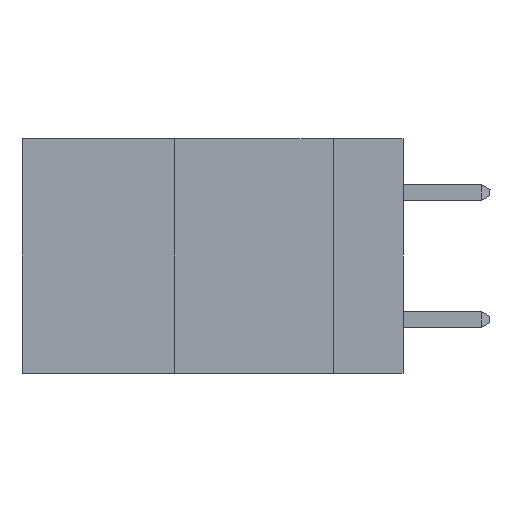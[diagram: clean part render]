
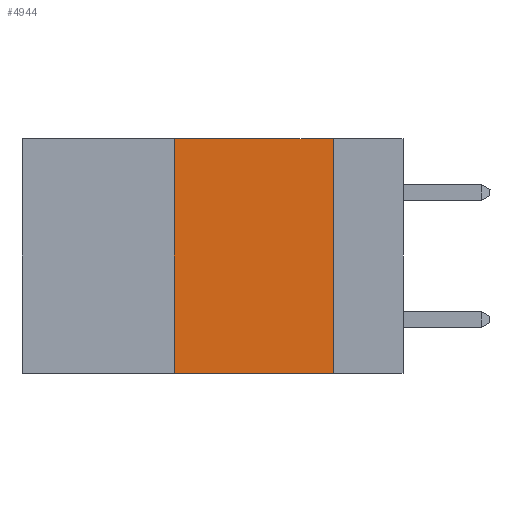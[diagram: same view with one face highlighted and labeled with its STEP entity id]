
A CAD part, left-side view. The second image highlights one B-rep face of the part: STEP entity #4944.
In plain terms, the highlighted planar face has unit normal (-1, 0, 0).
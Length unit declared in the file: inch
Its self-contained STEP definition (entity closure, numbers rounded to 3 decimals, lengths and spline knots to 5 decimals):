
#796 = VERTEX_POINT ( 'NONE', #2833 ) ;
#2022 = VERTEX_POINT ( 'NONE', #2783 ) ;
#2783 = CARTESIAN_POINT ( 'NONE',  ( 0., 0.36, 0. ) ) ;
#2833 = CARTESIAN_POINT ( 'NONE',  ( 0., 0.36, -0.37 ) ) ;
#4078 = VERTEX_POINT ( 'NONE', #7109 ) ;
#4373 = ORIENTED_EDGE ( 'NONE', *, *, #6924, .F. ) ;
#4425 = EDGE_LOOP ( 'NONE', ( #4373, #6358, #9273, #11329 ) ) ;
#4778 = PLANE ( 'NONE',  #5179 ) ;
#4801 = LINE ( 'NONE', #6913, #13513 ) ;
#4944 = ADVANCED_FACE ( 'NONE', ( #5834 ), #4778, .F. ) ;
#5179 = AXIS2_PLACEMENT_3D ( 'NONE', #8188, #6694, #9816 ) ;
#5188 = VECTOR ( 'NONE', #10470, 39.37008 ) ;
#5401 = EDGE_CURVE ( 'NONE', #796, #2022, #10566, .T. ) ;
#5834 = FACE_OUTER_BOUND ( 'NONE', #4425, .T. ) ;
#5972 = DIRECTION ( 'NONE',  ( 0., -1., 0. ) ) ;
#6358 = ORIENTED_EDGE ( 'NONE', *, *, #10787, .F. ) ;
#6694 = DIRECTION ( 'NONE',  ( 1., 0., 0. ) ) ;
#6913 = CARTESIAN_POINT ( 'NONE',  ( 0., 0.6, 0. ) ) ;
#6924 = EDGE_CURVE ( 'NONE', #7158, #4078, #13030, .T. ) ;
#7109 = CARTESIAN_POINT ( 'NONE',  ( 0., 0.11, -0.37 ) ) ;
#7158 = VERTEX_POINT ( 'NONE', #9756 ) ;
#7349 = VECTOR ( 'NONE', #9837, 39.37008 ) ;
#8188 = CARTESIAN_POINT ( 'NONE',  ( 0., 0.6, 0. ) ) ;
#8924 = EDGE_CURVE ( 'NONE', #796, #4078, #11851, .T. ) ;
#9180 = VECTOR ( 'NONE', #11585, 39.37008 ) ;
#9273 = ORIENTED_EDGE ( 'NONE', *, *, #5401, .F. ) ;
#9756 = CARTESIAN_POINT ( 'NONE',  ( 0., 0.11, 0. ) ) ;
#9816 = DIRECTION ( 'NONE',  ( 0., 0., -1. ) ) ;
#9837 = DIRECTION ( 'NONE',  ( 0., 0., -1. ) ) ;
#10190 = CARTESIAN_POINT ( 'NONE',  ( 0., 0.11, 0. ) ) ;
#10470 = DIRECTION ( 'NONE',  ( 0., 0., 1. ) ) ;
#10566 = LINE ( 'NONE', #11954, #5188 ) ;
#10591 = CARTESIAN_POINT ( 'NONE',  ( 0., 0.6, -0.37 ) ) ;
#10787 = EDGE_CURVE ( 'NONE', #2022, #7158, #4801, .T. ) ;
#11329 = ORIENTED_EDGE ( 'NONE', *, *, #8924, .T. ) ;
#11585 = DIRECTION ( 'NONE',  ( 0., -1., 0. ) ) ;
#11851 = LINE ( 'NONE', #10591, #9180 ) ;
#11954 = CARTESIAN_POINT ( 'NONE',  ( 0., 0.36, 0. ) ) ;
#13030 = LINE ( 'NONE', #10190, #7349 ) ;
#13513 = VECTOR ( 'NONE', #5972, 39.37008 ) ;
